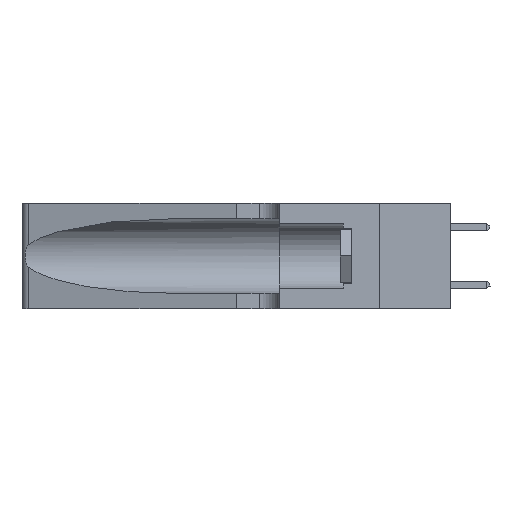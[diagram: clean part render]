
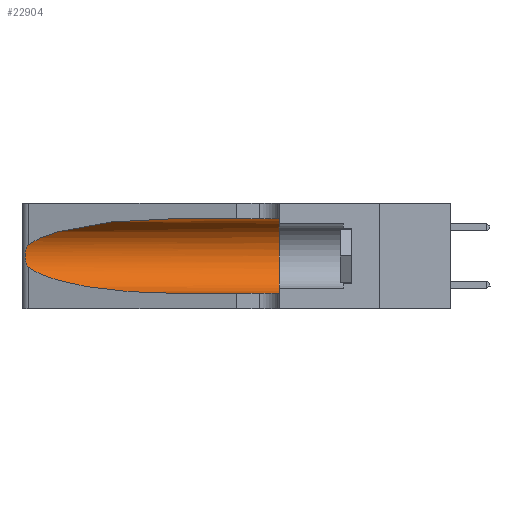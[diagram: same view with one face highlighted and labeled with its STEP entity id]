
A CAD part, left-side view. The second image highlights one B-rep face of the part: STEP entity #22904.
In plain terms, the highlighted cylindrical face has radius 3.308 mm (diameter 6.617 mm), a partial arc.
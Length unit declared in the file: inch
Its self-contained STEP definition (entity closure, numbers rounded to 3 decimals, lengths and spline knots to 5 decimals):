
#696 = CARTESIAN_POINT ( 'NONE',  ( 0.25555, 1.22994, 0.2215 ) ) ;
#1012 = CARTESIAN_POINT ( 'NONE',  ( 0.25555, 1.22993, 0.14849 ) ) ;
#1282 = CARTESIAN_POINT ( 'NONE',  ( 0.2373, 1.15595, 0.08982 ) ) ;
#1401 = EDGE_CURVE ( 'NONE', #44986, #8058, #35467, .T. ) ;
#2583 = CARTESIAN_POINT ( 'NONE',  ( 0.1305, 0.72297, 0.05475 ) ) ;
#2636 = CARTESIAN_POINT ( 'NONE',  ( 0.1305, 1.61858, 0.31525 ) ) ;
#3117 = AXIS2_PLACEMENT_3D ( 'NONE', #18859, #43781, #22469 ) ;
#3337 = ORIENTED_EDGE ( 'NONE', *, *, #37868, .T. ) ;
#5034 = CARTESIAN_POINT ( 'NONE',  ( 0.1305, 0.35, 0.05475 ) ) ;
#5382 = LINE ( 'NONE', #2636, #24440 ) ;
#5612 = ORIENTED_EDGE ( 'NONE', *, *, #23096, .T. ) ;
#6588 = CARTESIAN_POINT ( 'NONE',  ( 0.1305, 0.72297, 0.31525 ) ) ;
#7086 =( BOUNDED_CURVE ( )  B_SPLINE_CURVE ( 3, ( #22715, #1282, #33514, #12108 ),
 .UNSPECIFIED., .F., .F. ) 
 B_SPLINE_CURVE_WITH_KNOTS ( ( 4, 4 ),
 ( 3.44316, 4.71239 ),
 .UNSPECIFIED. ) 
 CURVE ( )  GEOMETRIC_REPRESENTATION_ITEM ( )  RATIONAL_B_SPLINE_CURVE ( ( 1., 0.87, 0.87, 1. ) ) 
 REPRESENTATION_ITEM ( '' )  );
#8048 = CARTESIAN_POINT ( 'NONE',  ( 0.25787, 1.23484, 0.2124 ) ) ;
#8058 = VERTEX_POINT ( 'NONE', #13396 ) ;
#10746 = VECTOR ( 'NONE', #38118, 39.37008 ) ;
#10951 = EDGE_LOOP ( 'NONE', ( #45836, #5612, #31675, #3337, #18430, #40602 ) ) ;
#11002 = CIRCLE ( 'NONE', #3117, 0.13025 ) ;
#11667 = CARTESIAN_POINT ( 'NONE',  ( 0.26018, 1.23835, 0.19895 ) ) ;
#12108 = CARTESIAN_POINT ( 'NONE',  ( 0.1305, 0.72297, 0.05475 ) ) ;
#13396 = CARTESIAN_POINT ( 'NONE',  ( 0.25487, 1.22718, 0.22369 ) ) ;
#13646 = CARTESIAN_POINT ( 'NONE',  ( 0.2373, 1.15595, 0.28018 ) ) ;
#15249 = CARTESIAN_POINT ( 'NONE',  ( 0.26075, 1.23896, 0.178 ) ) ;
#15403 = B_SPLINE_CURVE_WITH_KNOTS ( 'NONE', 3,
 ( #25929, #696, #29546, #8048, #33090, #11667, #36621, #15249, #40188, #18850, #43773, #22456, #1012, #26086 ),
 .UNSPECIFIED., .F., .F.,
 ( 4, 2, 2, 2, 2, 2, 4 ),
 ( 0., 0.00027, 0.00053, 0.00107, 0.0016, 0.00187, 0.00214 ),
 .UNSPECIFIED. ) ;
#16676 = DIRECTION ( 'NONE',  ( 0., 0., -1. ) ) ;
#18231 = EDGE_CURVE ( 'NONE', #44986, #19074, #5382, .T. ) ;
#18430 = ORIENTED_EDGE ( 'NONE', *, *, #34531, .F. ) ;
#18850 = CARTESIAN_POINT ( 'NONE',  ( 0.25856, 1.23593, 0.16098 ) ) ;
#18859 = CARTESIAN_POINT ( 'NONE',  ( 0.1305, 0.35, 0.185 ) ) ;
#19074 = VERTEX_POINT ( 'NONE', #20152 ) ;
#19136 = LINE ( 'NONE', #34598, #10746 ) ;
#20152 = CARTESIAN_POINT ( 'NONE',  ( 0.1305, 0.35, 0.31525 ) ) ;
#20264 = CARTESIAN_POINT ( 'NONE',  ( 0.1305, 1.61858, 0.185 ) ) ;
#22456 = CARTESIAN_POINT ( 'NONE',  ( 0.25639, 1.23186, 0.15144 ) ) ;
#22469 = DIRECTION ( 'NONE',  ( 0., 0., 1. ) ) ;
#22715 = CARTESIAN_POINT ( 'NONE',  ( 0.25487, 1.22718, 0.14631 ) ) ;
#22904 = ADVANCED_FACE ( 'NONE', ( #34461 ), #32256, .F. ) ;
#23096 = EDGE_CURVE ( 'NONE', #8058, #24371, #15403, .T. ) ;
#24064 = DIRECTION ( 'NONE',  ( 0., -1., 0. ) ) ;
#24371 = VERTEX_POINT ( 'NONE', #43062 ) ;
#24440 = VECTOR ( 'NONE', #24064, 39.37008 ) ;
#24699 = DIRECTION ( 'NONE',  ( 0., -1., 0. ) ) ;
#25929 = CARTESIAN_POINT ( 'NONE',  ( 0.25487, 1.22718, 0.22369 ) ) ;
#26086 = CARTESIAN_POINT ( 'NONE',  ( 0.25487, 1.22718, 0.14631 ) ) ;
#26585 = CARTESIAN_POINT ( 'NONE',  ( 0.1305, 0.72297, 0.31525 ) ) ;
#27544 = AXIS2_PLACEMENT_3D ( 'NONE', #20264, #24699, #16676 ) ;
#29546 = CARTESIAN_POINT ( 'NONE',  ( 0.25639, 1.23184, 0.21858 ) ) ;
#29962 = EDGE_CURVE ( 'NONE', #24371, #34862, #7086, .T. ) ;
#31640 = CARTESIAN_POINT ( 'NONE',  ( 0.25487, 1.22718, 0.22369 ) ) ;
#31675 = ORIENTED_EDGE ( 'NONE', *, *, #29962, .T. ) ;
#32256 = CYLINDRICAL_SURFACE ( 'NONE', #27544, 0.13025 ) ;
#33090 = CARTESIAN_POINT ( 'NONE',  ( 0.25854, 1.2359, 0.20912 ) ) ;
#33514 = CARTESIAN_POINT ( 'NONE',  ( 0.18966, 0.96281, 0.05475 ) ) ;
#34461 = FACE_OUTER_BOUND ( 'NONE', #10951, .T. ) ;
#34531 = EDGE_CURVE ( 'NONE', #19074, #42717, #11002, .T. ) ;
#34598 = CARTESIAN_POINT ( 'NONE',  ( 0.1305, 1.61858, 0.05475 ) ) ;
#34862 = VERTEX_POINT ( 'NONE', #2583 ) ;
#35467 =( BOUNDED_CURVE ( )  B_SPLINE_CURVE ( 3, ( #6588, #42145, #13646, #31640 ),
 .UNSPECIFIED., .F., .T. ) 
 B_SPLINE_CURVE_WITH_KNOTS ( ( 4, 4 ),
 ( 1.5708, 2.84003 ),
 .UNSPECIFIED. ) 
 CURVE ( )  GEOMETRIC_REPRESENTATION_ITEM ( )  RATIONAL_B_SPLINE_CURVE ( ( 1., 0.87, 0.87, 1. ) ) 
 REPRESENTATION_ITEM ( '' )  );
#36621 = CARTESIAN_POINT ( 'NONE',  ( 0.26075, 1.23896, 0.19203 ) ) ;
#37868 = EDGE_CURVE ( 'NONE', #34862, #42717, #19136, .T. ) ;
#38118 = DIRECTION ( 'NONE',  ( 0., -1., 0. ) ) ;
#40188 = CARTESIAN_POINT ( 'NONE',  ( 0.26017, 1.23833, 0.17102 ) ) ;
#40602 = ORIENTED_EDGE ( 'NONE', *, *, #18231, .F. ) ;
#42145 = CARTESIAN_POINT ( 'NONE',  ( 0.18966, 0.96281, 0.31525 ) ) ;
#42717 = VERTEX_POINT ( 'NONE', #5034 ) ;
#43062 = CARTESIAN_POINT ( 'NONE',  ( 0.25487, 1.22718, 0.14631 ) ) ;
#43773 = CARTESIAN_POINT ( 'NONE',  ( 0.25789, 1.23486, 0.15765 ) ) ;
#43781 = DIRECTION ( 'NONE',  ( 0., 1., 0. ) ) ;
#44986 = VERTEX_POINT ( 'NONE', #26585 ) ;
#45836 = ORIENTED_EDGE ( 'NONE', *, *, #1401, .T. ) ;
